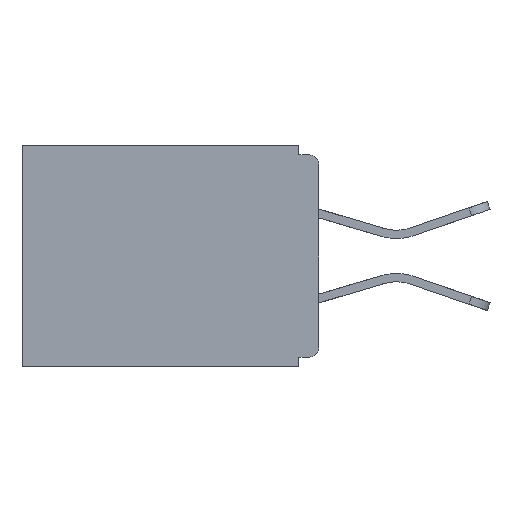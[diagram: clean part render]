
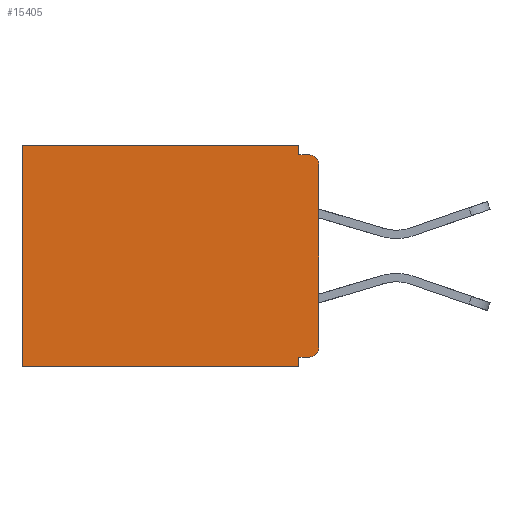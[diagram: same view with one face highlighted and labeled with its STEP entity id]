
A CAD part, left-side view. The second image highlights one B-rep face of the part: STEP entity #15405.
In plain terms, the highlighted planar face has unit normal (-1, 0, 0).
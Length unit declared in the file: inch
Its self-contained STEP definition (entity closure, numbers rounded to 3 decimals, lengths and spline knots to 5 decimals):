
#252 = VERTEX_POINT ( 'NONE', #2021 ) ;
#352 = CARTESIAN_POINT ( 'NONE',  ( 0.298, 0.031, -0.328 ) ) ;
#441 = DIRECTION ( 'NONE',  ( 0., 1., 0. ) ) ;
#581 = DIRECTION ( 'NONE',  ( 0., -1., 0. ) ) ;
#1071 = DIRECTION ( 'NONE',  ( 0., 0., -1. ) ) ;
#1787 = DIRECTION ( 'NONE',  ( 0., 0., -1. ) ) ;
#1819 = VECTOR ( 'NONE', #441, 39.37008 ) ;
#2021 = CARTESIAN_POINT ( 'NONE',  ( 0.298, 0.031, 0. ) ) ;
#2293 = CARTESIAN_POINT ( 'NONE',  ( 0.298, 0., 0. ) ) ;
#2606 = LINE ( 'NONE', #2293, #20178 ) ;
#3779 = DIRECTION ( 'NONE',  ( 0., 0., -1. ) ) ;
#4144 = VECTOR ( 'NONE', #1071, 39.37008 ) ;
#4547 = DIRECTION ( 'NONE',  ( 0., 0., -1. ) ) ;
#4616 = ORIENTED_EDGE ( 'NONE', *, *, #24937, .F. ) ;
#4985 = EDGE_CURVE ( 'NONE', #22561, #17919, #17197, .T. ) ;
#5084 = AXIS2_PLACEMENT_3D ( 'NONE', #12033, #5773, #1787 ) ;
#5093 = LINE ( 'NONE', #19949, #11316 ) ;
#5762 = CARTESIAN_POINT ( 'NONE',  ( 0.298, 0., -0.313 ) ) ;
#5773 = DIRECTION ( 'NONE',  ( -1., 0., 0. ) ) ;
#6751 = EDGE_CURVE ( 'NONE', #24891, #8822, #22091, .T. ) ;
#7866 = DIRECTION ( 'NONE',  ( -1., 0., 0. ) ) ;
#8026 = LINE ( 'NONE', #16283, #1819 ) ;
#8179 = VERTEX_POINT ( 'NONE', #17544 ) ;
#8182 = DIRECTION ( 'NONE',  ( 0., 0., -1. ) ) ;
#8314 = VECTOR ( 'NONE', #12278, 39.37008 ) ;
#8364 = VERTEX_POINT ( 'NONE', #352 ) ;
#8587 = CARTESIAN_POINT ( 'NONE',  ( 0.298, 0.015, -0.328 ) ) ;
#8822 = VERTEX_POINT ( 'NONE', #5762 ) ;
#9745 = DIRECTION ( 'NONE',  ( 0., 0., -1. ) ) ;
#9752 = ORIENTED_EDGE ( 'NONE', *, *, #13120, .F. ) ;
#10149 = DIRECTION ( 'NONE',  ( 0., 1., 0. ) ) ;
#10505 = CARTESIAN_POINT ( 'NONE',  ( 0.298, 0.031, -0.343 ) ) ;
#10778 = VERTEX_POINT ( 'NONE', #23781 ) ;
#10828 = LINE ( 'NONE', #10505, #15750 ) ;
#11053 = CARTESIAN_POINT ( 'NONE',  ( 0.298, 0.46, 0. ) ) ;
#11288 = VECTOR ( 'NONE', #581, 39.37008 ) ;
#11316 = VECTOR ( 'NONE', #8182, 39.37008 ) ;
#11416 = ORIENTED_EDGE ( 'NONE', *, *, #22033, .F. ) ;
#12033 = CARTESIAN_POINT ( 'NONE',  ( 0.298, 0.015, -0.313 ) ) ;
#12278 = DIRECTION ( 'NONE',  ( 0., 1., 0. ) ) ;
#12462 = EDGE_CURVE ( 'NONE', #8364, #10778, #5093, .T. ) ;
#12714 = VERTEX_POINT ( 'NONE', #17561 ) ;
#13120 = EDGE_CURVE ( 'NONE', #22561, #8822, #2606, .T. ) ;
#13249 = LINE ( 'NONE', #23797, #8314 ) ;
#13477 = CARTESIAN_POINT ( 'NONE',  ( 0.298, 0., 0. ) ) ;
#13570 = EDGE_CURVE ( 'NONE', #12714, #8179, #21089, .T. ) ;
#14044 = CARTESIAN_POINT ( 'NONE',  ( 0.298, 0., -0.328 ) ) ;
#14680 = AXIS2_PLACEMENT_3D ( 'NONE', #23913, #7866, #3779 ) ;
#15405 = ADVANCED_FACE ( 'NONE', ( #25337 ), #23012, .F. ) ;
#15654 = LINE ( 'NONE', #14044, #23028 ) ;
#15750 = VECTOR ( 'NONE', #22118, 39.37008 ) ;
#16283 = CARTESIAN_POINT ( 'NONE',  ( 0.298, 0., 0. ) ) ;
#16451 = ORIENTED_EDGE ( 'NONE', *, *, #23779, .F. ) ;
#16657 = ORIENTED_EDGE ( 'NONE', *, *, #4985, .T. ) ;
#16868 = ORIENTED_EDGE ( 'NONE', *, *, #12462, .F. ) ;
#16946 = ORIENTED_EDGE ( 'NONE', *, *, #18359, .F. ) ;
#17197 = CIRCLE ( 'NONE', #14680, 0.015 ) ;
#17544 = CARTESIAN_POINT ( 'NONE',  ( 0.298, 0.46, -0.343 ) ) ;
#17561 = CARTESIAN_POINT ( 'NONE',  ( 0.298, 0.46, 0. ) ) ;
#17919 = VERTEX_POINT ( 'NONE', #22435 ) ;
#18359 = EDGE_CURVE ( 'NONE', #10778, #8179, #13249, .T. ) ;
#18950 = LINE ( 'NONE', #24356, #11288 ) ;
#19949 = CARTESIAN_POINT ( 'NONE',  ( 0.298, 0.031, -0.343 ) ) ;
#20178 = VECTOR ( 'NONE', #4547, 39.37008 ) ;
#20984 = VERTEX_POINT ( 'NONE', #22312 ) ;
#21089 = LINE ( 'NONE', #11053, #4144 ) ;
#21302 = ORIENTED_EDGE ( 'NONE', *, *, #6751, .T. ) ;
#21782 = DIRECTION ( 'NONE',  ( 1., 0., 0. ) ) ;
#21886 = AXIS2_PLACEMENT_3D ( 'NONE', #13477, #21782, #9745 ) ;
#22033 = EDGE_CURVE ( 'NONE', #252, #20984, #10828, .T. ) ;
#22091 = CIRCLE ( 'NONE', #5084, 0.015 ) ;
#22118 = DIRECTION ( 'NONE',  ( 0., 0., -1. ) ) ;
#22260 = CARTESIAN_POINT ( 'NONE',  ( 0.298, 0., -0.03 ) ) ;
#22299 = EDGE_CURVE ( 'NONE', #252, #12714, #8026, .T. ) ;
#22312 = CARTESIAN_POINT ( 'NONE',  ( 0.298, 0.031, -0.015 ) ) ;
#22435 = CARTESIAN_POINT ( 'NONE',  ( 0.298, 0.015, -0.015 ) ) ;
#22561 = VERTEX_POINT ( 'NONE', #22260 ) ;
#23012 = PLANE ( 'NONE',  #21886 ) ;
#23028 = VECTOR ( 'NONE', #10149, 39.37008 ) ;
#23779 = EDGE_CURVE ( 'NONE', #24891, #8364, #15654, .T. ) ;
#23781 = CARTESIAN_POINT ( 'NONE',  ( 0.298, 0.031, -0.343 ) ) ;
#23797 = CARTESIAN_POINT ( 'NONE',  ( 0.298, 0., -0.343 ) ) ;
#23913 = CARTESIAN_POINT ( 'NONE',  ( 0.298, 0.015, -0.03 ) ) ;
#23949 = EDGE_LOOP ( 'NONE', ( #16657, #4616, #11416, #24506, #24616, #16946, #16868, #16451, #21302, #9752 ) ) ;
#24356 = CARTESIAN_POINT ( 'NONE',  ( 0.298, 0., -0.015 ) ) ;
#24506 = ORIENTED_EDGE ( 'NONE', *, *, #22299, .T. ) ;
#24616 = ORIENTED_EDGE ( 'NONE', *, *, #13570, .T. ) ;
#24891 = VERTEX_POINT ( 'NONE', #8587 ) ;
#24937 = EDGE_CURVE ( 'NONE', #20984, #17919, #18950, .T. ) ;
#25337 = FACE_OUTER_BOUND ( 'NONE', #23949, .T. ) ;
